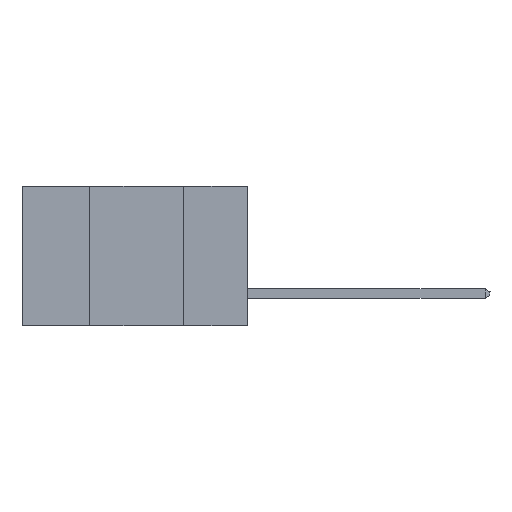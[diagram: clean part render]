
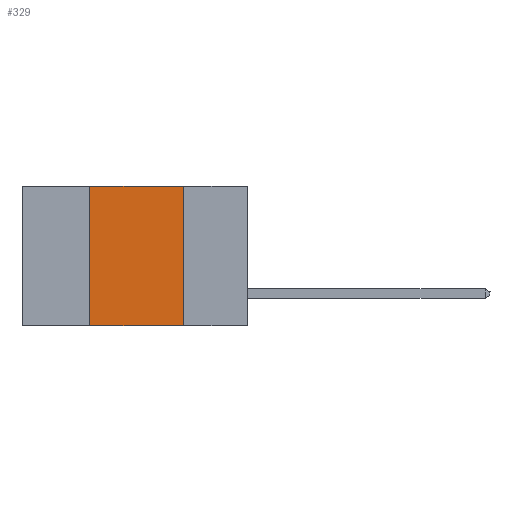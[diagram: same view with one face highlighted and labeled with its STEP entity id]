
A CAD part, left-side view. The second image highlights one B-rep face of the part: STEP entity #329.
In plain terms, the highlighted planar face has unit normal (-1, 0, 0).
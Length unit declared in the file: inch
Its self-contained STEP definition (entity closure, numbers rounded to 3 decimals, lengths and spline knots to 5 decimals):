
#329 = ADVANCED_FACE ( 'NONE', ( #11924 ), #6203, .F. ) ;
#338 = CARTESIAN_POINT ( 'NONE',  ( 0., 0.17, -0.37 ) ) ;
#385 = EDGE_CURVE ( 'NONE', #1597, #7816, #10154, .T. ) ;
#1597 = VERTEX_POINT ( 'NONE', #9681 ) ;
#1913 = ORIENTED_EDGE ( 'NONE', *, *, #4759, .F. ) ;
#2006 = ORIENTED_EDGE ( 'NONE', *, *, #10583, .T. ) ;
#2105 = DIRECTION ( 'NONE',  ( 0., 0., 1. ) ) ;
#3269 = CARTESIAN_POINT ( 'NONE',  ( 0., 0.42, -0.37 ) ) ;
#3437 = DIRECTION ( 'NONE',  ( 0., 0., -1. ) ) ;
#3474 = AXIS2_PLACEMENT_3D ( 'NONE', #11004, #5230, #10941 ) ;
#4759 = EDGE_CURVE ( 'NONE', #5667, #8805, #10252, .T. ) ;
#4941 = VECTOR ( 'NONE', #2105, 39.37008 ) ;
#5039 = CARTESIAN_POINT ( 'NONE',  ( 0., 0.6, -0.37 ) ) ;
#5230 = DIRECTION ( 'NONE',  ( 1., 0., 0. ) ) ;
#5456 = CARTESIAN_POINT ( 'NONE',  ( 0., 0.17, 0. ) ) ;
#5667 = VERTEX_POINT ( 'NONE', #5456 ) ;
#5925 = ORIENTED_EDGE ( 'NONE', *, *, #385, .F. ) ;
#6203 = PLANE ( 'NONE',  #3474 ) ;
#6623 = LINE ( 'NONE', #10449, #8832 ) ;
#6747 = CARTESIAN_POINT ( 'NONE',  ( 0., 0.42, 0. ) ) ;
#7816 = VERTEX_POINT ( 'NONE', #6747 ) ;
#7938 = DIRECTION ( 'NONE',  ( 0., -1., 0. ) ) ;
#8631 = ORIENTED_EDGE ( 'NONE', *, *, #8801, .F. ) ;
#8801 = EDGE_CURVE ( 'NONE', #7816, #5667, #6623, .T. ) ;
#8805 = VERTEX_POINT ( 'NONE', #12616 ) ;
#8832 = VECTOR ( 'NONE', #12409, 39.37008 ) ;
#9097 = EDGE_LOOP ( 'NONE', ( #1913, #8631, #5925, #2006 ) ) ;
#9681 = CARTESIAN_POINT ( 'NONE',  ( 0., 0.42, -0.37 ) ) ;
#9692 = VECTOR ( 'NONE', #7938, 39.37008 ) ;
#9797 = VECTOR ( 'NONE', #3437, 39.37008 ) ;
#10154 = LINE ( 'NONE', #3269, #4941 ) ;
#10252 = LINE ( 'NONE', #338, #9797 ) ;
#10449 = CARTESIAN_POINT ( 'NONE',  ( 0., 0.6, 0. ) ) ;
#10583 = EDGE_CURVE ( 'NONE', #1597, #8805, #11071, .T. ) ;
#10941 = DIRECTION ( 'NONE',  ( 0., 0., -1. ) ) ;
#11004 = CARTESIAN_POINT ( 'NONE',  ( 0., 0.6, 0. ) ) ;
#11071 = LINE ( 'NONE', #5039, #9692 ) ;
#11924 = FACE_OUTER_BOUND ( 'NONE', #9097, .T. ) ;
#12409 = DIRECTION ( 'NONE',  ( 0., -1., 0. ) ) ;
#12616 = CARTESIAN_POINT ( 'NONE',  ( 0., 0.17, -0.37 ) ) ;
